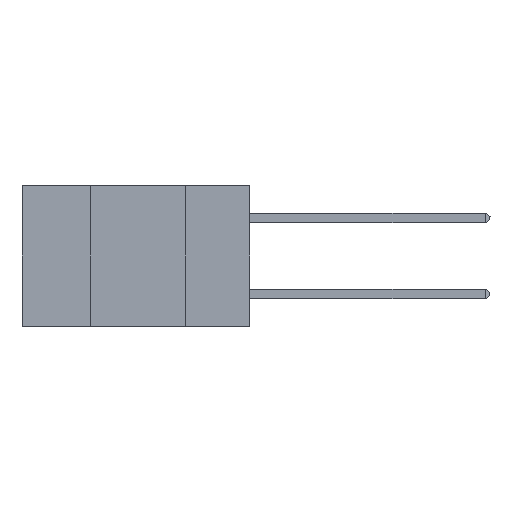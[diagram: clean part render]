
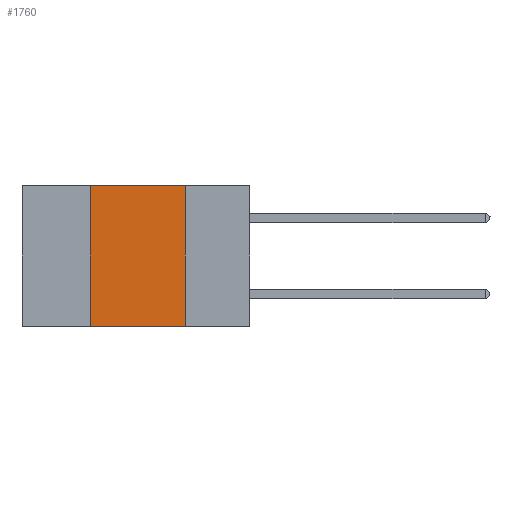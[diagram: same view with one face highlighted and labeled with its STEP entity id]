
A CAD part, left-side view. The second image highlights one B-rep face of the part: STEP entity #1760.
In plain terms, the highlighted planar face has unit normal (-1, 0, 0).
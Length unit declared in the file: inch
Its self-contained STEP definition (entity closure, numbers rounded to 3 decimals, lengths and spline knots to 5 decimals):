
#120 = ORIENTED_EDGE ( 'NONE', *, *, #2502, .F. ) ;
#1760 = ADVANCED_FACE ( 'NONE', ( #27291 ), #19053, .F. ) ;
#2415 = EDGE_CURVE ( 'NONE', #17520, #6250, #12711, .T. ) ;
#2502 = EDGE_CURVE ( 'NONE', #17695, #17520, #8564, .T. ) ;
#6250 = VERTEX_POINT ( 'NONE', #11889 ) ;
#6923 = CARTESIAN_POINT ( 'NONE',  ( 0., 0.42, 0. ) ) ;
#7348 = DIRECTION ( 'NONE',  ( 0., 0., -1. ) ) ;
#7839 = DIRECTION ( 'NONE',  ( 0., 0., -1. ) ) ;
#8010 = DIRECTION ( 'NONE',  ( 0., -1., 0. ) ) ;
#8050 = VECTOR ( 'NONE', #8010, 39.37008 ) ;
#8564 = LINE ( 'NONE', #6923, #13739 ) ;
#9046 = CARTESIAN_POINT ( 'NONE',  ( 0., 0.42, -0.37 ) ) ;
#9336 = ORIENTED_EDGE ( 'NONE', *, *, #2415, .F. ) ;
#10247 = CARTESIAN_POINT ( 'NONE',  ( 0., 0.6, 0. ) ) ;
#10966 = ORIENTED_EDGE ( 'NONE', *, *, #23530, .F. ) ;
#11791 = CARTESIAN_POINT ( 'NONE',  ( 0., 0.17, -0.37 ) ) ;
#11889 = CARTESIAN_POINT ( 'NONE',  ( 0., 0.17, 0. ) ) ;
#12039 = VECTOR ( 'NONE', #7348, 39.37008 ) ;
#12711 = LINE ( 'NONE', #17534, #26565 ) ;
#13290 = CARTESIAN_POINT ( 'NONE',  ( 0., 0.42, 0. ) ) ;
#13739 = VECTOR ( 'NONE', #22427, 39.37008 ) ;
#15947 = ORIENTED_EDGE ( 'NONE', *, *, #27148, .T. ) ;
#17520 = VERTEX_POINT ( 'NONE', #13290 ) ;
#17534 = CARTESIAN_POINT ( 'NONE',  ( 0., 0.6, 0. ) ) ;
#17695 = VERTEX_POINT ( 'NONE', #9046 ) ;
#19053 = PLANE ( 'NONE',  #19315 ) ;
#19284 = DIRECTION ( 'NONE',  ( 0., -1., 0. ) ) ;
#19315 = AXIS2_PLACEMENT_3D ( 'NONE', #10247, #27669, #7839 ) ;
#21950 = LINE ( 'NONE', #28205, #8050 ) ;
#22317 = EDGE_LOOP ( 'NONE', ( #10966, #9336, #120, #15947 ) ) ;
#22427 = DIRECTION ( 'NONE',  ( 0., 0., 1. ) ) ;
#23530 = EDGE_CURVE ( 'NONE', #6250, #25268, #23848, .T. ) ;
#23848 = LINE ( 'NONE', #25237, #12039 ) ;
#25237 = CARTESIAN_POINT ( 'NONE',  ( 0., 0.17, 0. ) ) ;
#25268 = VERTEX_POINT ( 'NONE', #11791 ) ;
#26565 = VECTOR ( 'NONE', #19284, 39.37008 ) ;
#27148 = EDGE_CURVE ( 'NONE', #17695, #25268, #21950, .T. ) ;
#27291 = FACE_OUTER_BOUND ( 'NONE', #22317, .T. ) ;
#27669 = DIRECTION ( 'NONE',  ( 1., 0., 0. ) ) ;
#28205 = CARTESIAN_POINT ( 'NONE',  ( 0., 0.6, -0.37 ) ) ;
